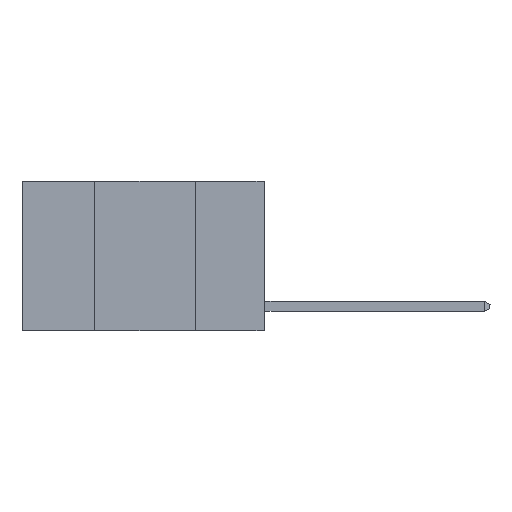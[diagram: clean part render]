
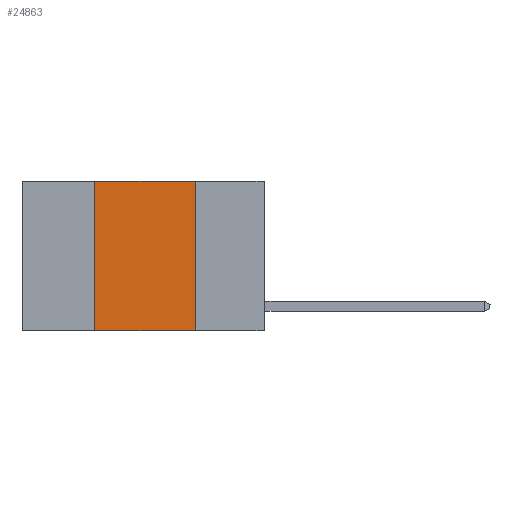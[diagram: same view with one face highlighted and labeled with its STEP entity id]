
A CAD part, left-side view. The second image highlights one B-rep face of the part: STEP entity #24863.
In plain terms, the highlighted planar face has unit normal (-1, 0, 0).
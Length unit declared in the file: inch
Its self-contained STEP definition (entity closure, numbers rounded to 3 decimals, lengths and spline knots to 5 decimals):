
#1023 = VECTOR ( 'NONE', #7142, 39.37008 ) ;
#1099 = LINE ( 'NONE', #9748, #1023 ) ;
#1544 = PLANE ( 'NONE',  #7363 ) ;
#1674 = FACE_OUTER_BOUND ( 'NONE', #9346, .T. ) ;
#3393 = DIRECTION ( 'NONE',  ( 0., 0., 1. ) ) ;
#3985 = LINE ( 'NONE', #19083, #19218 ) ;
#3998 = VERTEX_POINT ( 'NONE', #16432 ) ;
#4336 = LINE ( 'NONE', #16968, #25395 ) ;
#5079 = VERTEX_POINT ( 'NONE', #22545 ) ;
#5128 = DIRECTION ( 'NONE',  ( 1., 0., 0. ) ) ;
#5924 = EDGE_CURVE ( 'NONE', #5079, #11613, #4336, .T. ) ;
#6166 = CARTESIAN_POINT ( 'NONE',  ( 0., 0.17, 0. ) ) ;
#7142 = DIRECTION ( 'NONE',  ( 0., -1., 0. ) ) ;
#7205 = DIRECTION ( 'NONE',  ( 0., 0., -1. ) ) ;
#7363 = AXIS2_PLACEMENT_3D ( 'NONE', #21629, #5128, #7205 ) ;
#7770 = CARTESIAN_POINT ( 'NONE',  ( 0., 0.42, 0. ) ) ;
#8963 = EDGE_CURVE ( 'NONE', #3998, #26783, #1099, .T. ) ;
#9346 = EDGE_LOOP ( 'NONE', ( #14230, #19897, #11949, #23630 ) ) ;
#9748 = CARTESIAN_POINT ( 'NONE',  ( 0., 0.6, -0.37 ) ) ;
#11613 = VERTEX_POINT ( 'NONE', #6166 ) ;
#11949 = ORIENTED_EDGE ( 'NONE', *, *, #23278, .F. ) ;
#12348 = DIRECTION ( 'NONE',  ( 0., 0., -1. ) ) ;
#12427 = DIRECTION ( 'NONE',  ( 0., -1., 0. ) ) ;
#13696 = LINE ( 'NONE', #7770, #22729 ) ;
#14230 = ORIENTED_EDGE ( 'NONE', *, *, #22842, .F. ) ;
#15501 = CARTESIAN_POINT ( 'NONE',  ( 0., 0.17, -0.37 ) ) ;
#16432 = CARTESIAN_POINT ( 'NONE',  ( 0., 0.42, -0.37 ) ) ;
#16968 = CARTESIAN_POINT ( 'NONE',  ( 0., 0.6, 0. ) ) ;
#19083 = CARTESIAN_POINT ( 'NONE',  ( 0., 0.17, 0. ) ) ;
#19218 = VECTOR ( 'NONE', #12348, 39.37008 ) ;
#19897 = ORIENTED_EDGE ( 'NONE', *, *, #5924, .F. ) ;
#21629 = CARTESIAN_POINT ( 'NONE',  ( 0., 0.6, 0. ) ) ;
#22545 = CARTESIAN_POINT ( 'NONE',  ( 0., 0.42, 0. ) ) ;
#22729 = VECTOR ( 'NONE', #3393, 39.37008 ) ;
#22842 = EDGE_CURVE ( 'NONE', #11613, #26783, #3985, .T. ) ;
#23278 = EDGE_CURVE ( 'NONE', #3998, #5079, #13696, .T. ) ;
#23630 = ORIENTED_EDGE ( 'NONE', *, *, #8963, .T. ) ;
#24863 = ADVANCED_FACE ( 'NONE', ( #1674 ), #1544, .F. ) ;
#25395 = VECTOR ( 'NONE', #12427, 39.37008 ) ;
#26783 = VERTEX_POINT ( 'NONE', #15501 ) ;
